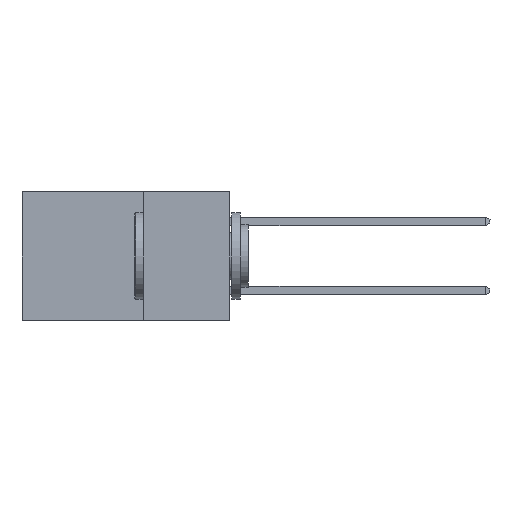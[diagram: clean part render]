
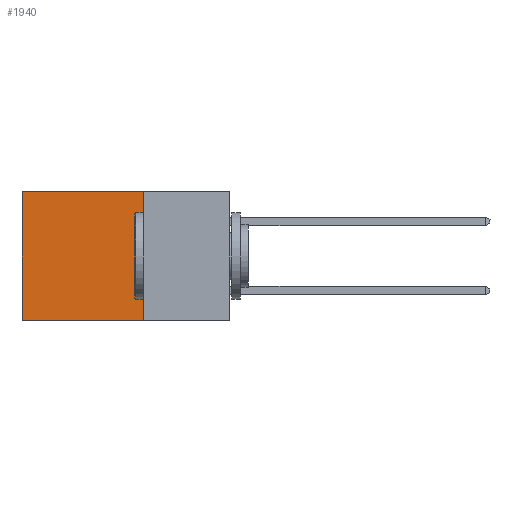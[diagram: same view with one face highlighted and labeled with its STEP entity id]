
A CAD part, left-side view. The second image highlights one B-rep face of the part: STEP entity #1940.
In plain terms, the highlighted planar face has unit normal (-1, 0, 0).
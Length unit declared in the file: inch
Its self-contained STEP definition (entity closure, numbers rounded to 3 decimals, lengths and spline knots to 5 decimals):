
#146 = CARTESIAN_POINT ( 'NONE',  ( 0.2615, 0.6, -0.37 ) ) ;
#269 = DIRECTION ( 'NONE',  ( 1., 0., 0. ) ) ;
#377 = LINE ( 'NONE', #7211, #3684 ) ;
#399 = EDGE_LOOP ( 'NONE', ( #3313, #3989, #1338, #4148 ) ) ;
#578 = VERTEX_POINT ( 'NONE', #2565 ) ;
#668 = CARTESIAN_POINT ( 'NONE',  ( 0.2615, 0.6, 0. ) ) ;
#753 = EDGE_CURVE ( 'NONE', #2161, #3529, #377, .T. ) ;
#1338 = ORIENTED_EDGE ( 'NONE', *, *, #8288, .F. ) ;
#1659 = CARTESIAN_POINT ( 'NONE',  ( 0.2615, 0.25, 0. ) ) ;
#1940 = ADVANCED_FACE ( 'NONE', ( #8054 ), #7839, .F. ) ;
#2161 = VERTEX_POINT ( 'NONE', #9325 ) ;
#2565 = CARTESIAN_POINT ( 'NONE',  ( 0.2615, 0.25, 0. ) ) ;
#2902 = VERTEX_POINT ( 'NONE', #668 ) ;
#3016 = EDGE_CURVE ( 'NONE', #2902, #3529, #6833, .T. ) ;
#3313 = ORIENTED_EDGE ( 'NONE', *, *, #3016, .T. ) ;
#3332 = LINE ( 'NONE', #10875, #8805 ) ;
#3529 = VERTEX_POINT ( 'NONE', #146 ) ;
#3589 = CARTESIAN_POINT ( 'NONE',  ( 0.2615, 0.25, -0.37 ) ) ;
#3684 = VECTOR ( 'NONE', #10610, 39.37008 ) ;
#3989 = ORIENTED_EDGE ( 'NONE', *, *, #753, .F. ) ;
#4148 = ORIENTED_EDGE ( 'NONE', *, *, #9946, .T. ) ;
#5089 = LINE ( 'NONE', #1659, #9525 ) ;
#5194 = DIRECTION ( 'NONE',  ( 0., 1., 0. ) ) ;
#5238 = VECTOR ( 'NONE', #6112, 39.37008 ) ;
#6112 = DIRECTION ( 'NONE',  ( 0., 0., -1. ) ) ;
#6833 = LINE ( 'NONE', #9391, #5238 ) ;
#7211 = CARTESIAN_POINT ( 'NONE',  ( 0.2615, 0.25, -0.37 ) ) ;
#7839 = PLANE ( 'NONE',  #10716 ) ;
#8054 = FACE_OUTER_BOUND ( 'NONE', #399, .T. ) ;
#8288 = EDGE_CURVE ( 'NONE', #578, #2161, #3332, .T. ) ;
#8317 = DIRECTION ( 'NONE',  ( 0., 0., -1. ) ) ;
#8724 = DIRECTION ( 'NONE',  ( 0., 0., -1. ) ) ;
#8805 = VECTOR ( 'NONE', #8317, 39.37008 ) ;
#9325 = CARTESIAN_POINT ( 'NONE',  ( 0.2615, 0.25, -0.37 ) ) ;
#9391 = CARTESIAN_POINT ( 'NONE',  ( 0.2615, 0.6, -0.37 ) ) ;
#9525 = VECTOR ( 'NONE', #5194, 39.37008 ) ;
#9946 = EDGE_CURVE ( 'NONE', #578, #2902, #5089, .T. ) ;
#10610 = DIRECTION ( 'NONE',  ( 0., 1., 0. ) ) ;
#10716 = AXIS2_PLACEMENT_3D ( 'NONE', #3589, #269, #8724 ) ;
#10875 = CARTESIAN_POINT ( 'NONE',  ( 0.2615, 0.25, -0.37 ) ) ;
